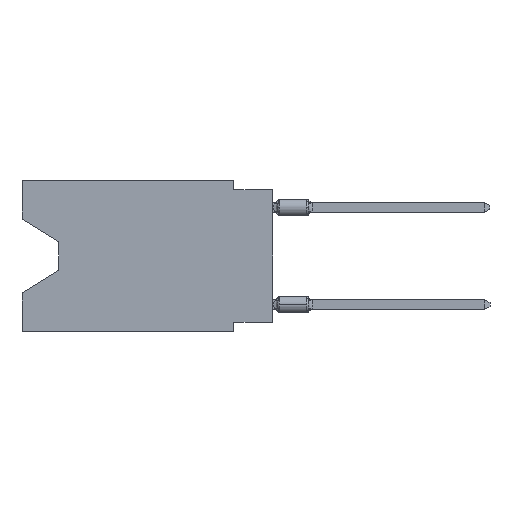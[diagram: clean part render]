
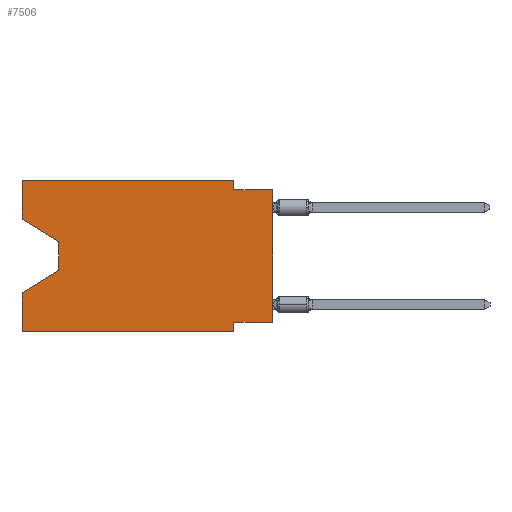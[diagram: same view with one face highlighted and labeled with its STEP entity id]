
A CAD part, left-side view. The second image highlights one B-rep face of the part: STEP entity #7506.
In plain terms, the highlighted planar face has unit normal (-1, 0, 0).
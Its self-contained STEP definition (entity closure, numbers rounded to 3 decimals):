
#283 = LINE ( 'NONE', #14993, #3051 ) ;
#380 = VECTOR ( 'NONE', #16667, 1000. ) ;
#419 = VERTEX_POINT ( 'NONE', #15826 ) ;
#422 = CARTESIAN_POINT ( 'NONE',  ( 0., 2.54, -0.635 ) ) ;
#769 = DIRECTION ( 'NONE',  ( 0., 0.855, -0.519 ) ) ;
#1757 = LINE ( 'NONE', #8660, #21259 ) ;
#1971 = DIRECTION ( 'NONE',  ( 0., -1., 0. ) ) ;
#2301 = VERTEX_POINT ( 'NONE', #6817 ) ;
#2354 = EDGE_CURVE ( 'NONE', #7500, #11521, #17086, .T. ) ;
#2610 = LINE ( 'NONE', #6265, #6433 ) ;
#2617 = EDGE_CURVE ( 'NONE', #18581, #20306, #6047, .T. ) ;
#3051 = VECTOR ( 'NONE', #18448, 1000. ) ;
#3348 = VECTOR ( 'NONE', #11237, 1000. ) ;
#3403 = EDGE_CURVE ( 'NONE', #20306, #419, #1757, .T. ) ;
#3504 = VECTOR ( 'NONE', #19460, 1000. ) ;
#3996 = DIRECTION ( 'NONE',  ( 0., 0., -1. ) ) ;
#4281 = CARTESIAN_POINT ( 'NONE',  ( 0., 2.54, -9.906 ) ) ;
#5018 = CARTESIAN_POINT ( 'NONE',  ( 0., 16.383, -9.906 ) ) ;
#5578 = EDGE_CURVE ( 'NONE', #13645, #13196, #6635, .T. ) ;
#5947 = VERTEX_POINT ( 'NONE', #8416 ) ;
#6047 = LINE ( 'NONE', #21295, #3348 ) ;
#6265 = CARTESIAN_POINT ( 'NONE',  ( 0., 13.97, -4.013 ) ) ;
#6343 = CARTESIAN_POINT ( 'NONE',  ( 0., 13.97, -5.893 ) ) ;
#6377 = EDGE_CURVE ( 'NONE', #6787, #7259, #11645, .T. ) ;
#6433 = VECTOR ( 'NONE', #19147, 1000. ) ;
#6635 = LINE ( 'NONE', #5018, #17053 ) ;
#6787 = VERTEX_POINT ( 'NONE', #19837 ) ;
#6817 = CARTESIAN_POINT ( 'NONE',  ( 0., 2.54, -9.271 ) ) ;
#6904 = ORIENTED_EDGE ( 'NONE', *, *, #19827, .F. ) ;
#7259 = VERTEX_POINT ( 'NONE', #13846 ) ;
#7321 = VECTOR ( 'NONE', #20468, 1000. ) ;
#7500 = VERTEX_POINT ( 'NONE', #6343 ) ;
#7506 = ADVANCED_FACE ( 'NONE', ( #11749 ), #19963, .F. ) ;
#7708 = ORIENTED_EDGE ( 'NONE', *, *, #16031, .F. ) ;
#8267 = ORIENTED_EDGE ( 'NONE', *, *, #13077, .F. ) ;
#8416 = CARTESIAN_POINT ( 'NONE',  ( 0., 13.97, -4.013 ) ) ;
#8462 = ORIENTED_EDGE ( 'NONE', *, *, #11202, .F. ) ;
#8484 = ORIENTED_EDGE ( 'NONE', *, *, #2617, .F. ) ;
#8543 = LINE ( 'NONE', #16761, #14224 ) ;
#8581 = EDGE_CURVE ( 'NONE', #5947, #7500, #2610, .T. ) ;
#8660 = CARTESIAN_POINT ( 'NONE',  ( 0., 16.383, 0. ) ) ;
#8971 = LINE ( 'NONE', #10704, #14864 ) ;
#9056 = CARTESIAN_POINT ( 'NONE',  ( 0., 16.383, -7.36 ) ) ;
#9609 = ORIENTED_EDGE ( 'NONE', *, *, #12128, .T. ) ;
#9758 = ORIENTED_EDGE ( 'NONE', *, *, #2354, .T. ) ;
#9815 = ORIENTED_EDGE ( 'NONE', *, *, #8581, .T. ) ;
#10014 = DIRECTION ( 'NONE',  ( 0., 0., -1. ) ) ;
#10232 = DIRECTION ( 'NONE',  ( 0., 0., 1. ) ) ;
#10246 = VECTOR ( 'NONE', #769, 1000. ) ;
#10353 = CARTESIAN_POINT ( 'NONE',  ( 0., 16.383, 0. ) ) ;
#10704 = CARTESIAN_POINT ( 'NONE',  ( 0., 0., -0.635 ) ) ;
#10913 = AXIS2_PLACEMENT_3D ( 'NONE', #20069, #18232, #10014 ) ;
#11202 = EDGE_CURVE ( 'NONE', #16182, #7259, #8971, .T. ) ;
#11237 = DIRECTION ( 'NONE',  ( 0., 0., 1. ) ) ;
#11521 = VERTEX_POINT ( 'NONE', #9056 ) ;
#11532 = ORIENTED_EDGE ( 'NONE', *, *, #6377, .T. ) ;
#11645 = LINE ( 'NONE', #16822, #14303 ) ;
#11749 = FACE_OUTER_BOUND ( 'NONE', #19077, .T. ) ;
#12128 = EDGE_CURVE ( 'NONE', #18581, #5947, #18280, .T. ) ;
#12863 = CARTESIAN_POINT ( 'NONE',  ( 0., 2.54, -9.906 ) ) ;
#13077 = EDGE_CURVE ( 'NONE', #13645, #11521, #283, .T. ) ;
#13196 = VERTEX_POINT ( 'NONE', #4281 ) ;
#13645 = VERTEX_POINT ( 'NONE', #19956 ) ;
#13752 = ORIENTED_EDGE ( 'NONE', *, *, #5578, .T. ) ;
#13846 = CARTESIAN_POINT ( 'NONE',  ( 0., 0., -0.635 ) ) ;
#14224 = VECTOR ( 'NONE', #3996, 1000. ) ;
#14303 = VECTOR ( 'NONE', #10232, 1000. ) ;
#14780 = ORIENTED_EDGE ( 'NONE', *, *, #18157, .F. ) ;
#14864 = VECTOR ( 'NONE', #20551, 1000. ) ;
#14993 = CARTESIAN_POINT ( 'NONE',  ( 0., 16.383, 0. ) ) ;
#15483 = LINE ( 'NONE', #17208, #7321 ) ;
#15700 = ORIENTED_EDGE ( 'NONE', *, *, #3403, .F. ) ;
#15826 = CARTESIAN_POINT ( 'NONE',  ( 0., 2.54, 0. ) ) ;
#16031 = EDGE_CURVE ( 'NONE', #2301, #13196, #17727, .T. ) ;
#16182 = VERTEX_POINT ( 'NONE', #422 ) ;
#16667 = DIRECTION ( 'NONE',  ( 0., -0.855, -0.519 ) ) ;
#16761 = CARTESIAN_POINT ( 'NONE',  ( 0., 2.54, 0. ) ) ;
#16822 = CARTESIAN_POINT ( 'NONE',  ( 0., 0., 0. ) ) ;
#17053 = VECTOR ( 'NONE', #18201, 1000. ) ;
#17056 = CARTESIAN_POINT ( 'NONE',  ( 0., 16.383, -2.546 ) ) ;
#17086 = LINE ( 'NONE', #20555, #10246 ) ;
#17208 = CARTESIAN_POINT ( 'NONE',  ( 0., 0., -9.271 ) ) ;
#17727 = LINE ( 'NONE', #12863, #3504 ) ;
#17962 = CARTESIAN_POINT ( 'NONE',  ( 0., 16.383, -2.546 ) ) ;
#18157 = EDGE_CURVE ( 'NONE', #6787, #2301, #15483, .T. ) ;
#18201 = DIRECTION ( 'NONE',  ( 0., -1., 0. ) ) ;
#18232 = DIRECTION ( 'NONE',  ( 1., 0., 0. ) ) ;
#18280 = LINE ( 'NONE', #17962, #380 ) ;
#18448 = DIRECTION ( 'NONE',  ( 0., 0., 1. ) ) ;
#18581 = VERTEX_POINT ( 'NONE', #17056 ) ;
#19077 = EDGE_LOOP ( 'NONE', ( #9609, #9815, #9758, #8267, #13752, #7708, #14780, #11532, #8462, #6904, #15700, #8484 ) ) ;
#19147 = DIRECTION ( 'NONE',  ( 0., 0., -1. ) ) ;
#19460 = DIRECTION ( 'NONE',  ( 0., 0., -1. ) ) ;
#19827 = EDGE_CURVE ( 'NONE', #419, #16182, #8543, .T. ) ;
#19837 = CARTESIAN_POINT ( 'NONE',  ( 0., 0., -9.271 ) ) ;
#19956 = CARTESIAN_POINT ( 'NONE',  ( 0., 16.383, -9.906 ) ) ;
#19963 = PLANE ( 'NONE',  #10913 ) ;
#20069 = CARTESIAN_POINT ( 'NONE',  ( 0., 16.383, 0. ) ) ;
#20306 = VERTEX_POINT ( 'NONE', #10353 ) ;
#20468 = DIRECTION ( 'NONE',  ( 0., 1., 0. ) ) ;
#20551 = DIRECTION ( 'NONE',  ( 0., -1., 0. ) ) ;
#20555 = CARTESIAN_POINT ( 'NONE',  ( 0., 13.97, -5.893 ) ) ;
#21259 = VECTOR ( 'NONE', #1971, 1000. ) ;
#21295 = CARTESIAN_POINT ( 'NONE',  ( 0., 16.383, 0. ) ) ;
